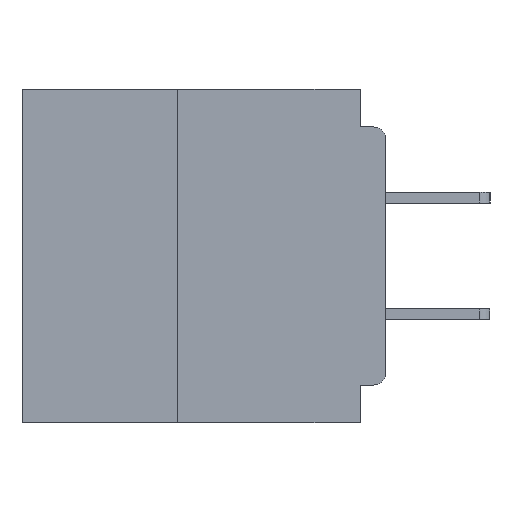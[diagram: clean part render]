
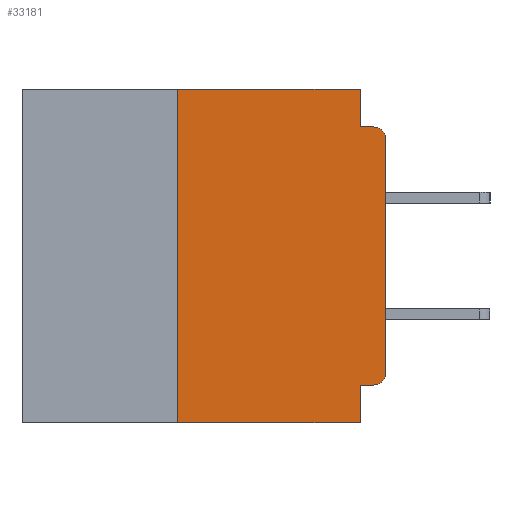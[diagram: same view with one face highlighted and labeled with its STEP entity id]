
A CAD part, left-side view. The second image highlights one B-rep face of the part: STEP entity #33181.
In plain terms, the highlighted planar face has unit normal (-1, 0, 0).
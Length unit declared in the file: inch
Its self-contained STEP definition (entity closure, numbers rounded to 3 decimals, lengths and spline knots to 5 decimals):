
#169 = CARTESIAN_POINT ( 'NONE',  ( 0., 0.437, 0. ) ) ;
#659 = CARTESIAN_POINT ( 'NONE',  ( 0., 0.015, -0.34 ) ) ;
#761 = ORIENTED_EDGE ( 'NONE', *, *, #18441, .F. ) ;
#800 = DIRECTION ( 'NONE',  ( 0., -1., 0. ) ) ;
#877 = VECTOR ( 'NONE', #6855, 39.37008 ) ;
#1191 = VECTOR ( 'NONE', #8662, 39.37008 ) ;
#1394 = LINE ( 'NONE', #33874, #30049 ) ;
#1563 = ORIENTED_EDGE ( 'NONE', *, *, #8156, .F. ) ;
#1566 = CARTESIAN_POINT ( 'NONE',  ( 0., 0.25, 0. ) ) ;
#2756 = CARTESIAN_POINT ( 'NONE',  ( 0., 0.031, 0. ) ) ;
#3075 = DIRECTION ( 'NONE',  ( 0., 0., -1. ) ) ;
#3431 = VECTOR ( 'NONE', #13379, 39.37008 ) ;
#3552 = DIRECTION ( 'NONE',  ( 0., 0., -1. ) ) ;
#4221 = VERTEX_POINT ( 'NONE', #32813 ) ;
#5037 = VERTEX_POINT ( 'NONE', #6826 ) ;
#5490 = CARTESIAN_POINT ( 'NONE',  ( 0., 0., -0.045 ) ) ;
#5972 = CARTESIAN_POINT ( 'NONE',  ( 0., 0.437, 0. ) ) ;
#6091 = DIRECTION ( 'NONE',  ( 0., -1., 0. ) ) ;
#6714 = LINE ( 'NONE', #35577, #28850 ) ;
#6826 = CARTESIAN_POINT ( 'NONE',  ( 0., 0., -0.34 ) ) ;
#6832 = ORIENTED_EDGE ( 'NONE', *, *, #22247, .T. ) ;
#6855 = DIRECTION ( 'NONE',  ( 0., 0., -1. ) ) ;
#7429 = CARTESIAN_POINT ( 'NONE',  ( 0., 0.015, -0.06 ) ) ;
#7729 = EDGE_LOOP ( 'NONE', ( #24704, #33731, #17093, #23660, #1563, #24869, #12643, #761, #22183, #6832 ) ) ;
#8156 = EDGE_CURVE ( 'NONE', #14080, #24318, #12377, .T. ) ;
#8567 = PLANE ( 'NONE',  #17278 ) ;
#8662 = DIRECTION ( 'NONE',  ( 0., 0., 1. ) ) ;
#9580 = CARTESIAN_POINT ( 'NONE',  ( 0., 0.031, -0.4 ) ) ;
#10043 = CARTESIAN_POINT ( 'NONE',  ( 0., 0.031, -0.4 ) ) ;
#10247 = DIRECTION ( 'NONE',  ( 0., 0., -1. ) ) ;
#11178 = CARTESIAN_POINT ( 'NONE',  ( 0., 0.015, -0.355 ) ) ;
#11506 = VERTEX_POINT ( 'NONE', #15536 ) ;
#11564 = VERTEX_POINT ( 'NONE', #26868 ) ;
#11615 = VECTOR ( 'NONE', #16721, 39.37008 ) ;
#12377 = LINE ( 'NONE', #5972, #18980 ) ;
#12612 = LINE ( 'NONE', #29885, #3431 ) ;
#12643 = ORIENTED_EDGE ( 'NONE', *, *, #27583, .T. ) ;
#13379 = DIRECTION ( 'NONE',  ( 0., 1., 0. ) ) ;
#13423 = VERTEX_POINT ( 'NONE', #10043 ) ;
#14080 = VERTEX_POINT ( 'NONE', #1566 ) ;
#15536 = CARTESIAN_POINT ( 'NONE',  ( 0., 0.031, -0.045 ) ) ;
#15836 = LINE ( 'NONE', #9580, #877 ) ;
#16721 = DIRECTION ( 'NONE',  ( 0., 0., -1. ) ) ;
#16782 = DIRECTION ( 'NONE',  ( 0., -1., 0. ) ) ;
#17027 = LINE ( 'NONE', #22579, #1191 ) ;
#17093 = ORIENTED_EDGE ( 'NONE', *, *, #17564, .F. ) ;
#17278 = AXIS2_PLACEMENT_3D ( 'NONE', #169, #19819, #3075 ) ;
#17564 = EDGE_CURVE ( 'NONE', #11506, #20044, #29651, .T. ) ;
#17688 = VERTEX_POINT ( 'NONE', #31086 ) ;
#17907 = CIRCLE ( 'NONE', #30913, 0.015 ) ;
#18441 = EDGE_CURVE ( 'NONE', #17688, #13423, #15836, .T. ) ;
#18980 = VECTOR ( 'NONE', #6091, 39.37008 ) ;
#19254 = CIRCLE ( 'NONE', #30952, 0.015 ) ;
#19414 = DIRECTION ( 'NONE',  ( 0., 0., 1. ) ) ;
#19819 = DIRECTION ( 'NONE',  ( 1., 0., 0. ) ) ;
#20044 = VERTEX_POINT ( 'NONE', #23678 ) ;
#20281 = DIRECTION ( 'NONE',  ( -1., 0., 0. ) ) ;
#20860 = CARTESIAN_POINT ( 'NONE',  ( 0., 0.031, 0. ) ) ;
#22183 = ORIENTED_EDGE ( 'NONE', *, *, #34793, .F. ) ;
#22247 = EDGE_CURVE ( 'NONE', #31831, #5037, #19254, .T. ) ;
#22579 = CARTESIAN_POINT ( 'NONE',  ( 0., 0., 0. ) ) ;
#23660 = ORIENTED_EDGE ( 'NONE', *, *, #30603, .F. ) ;
#23678 = CARTESIAN_POINT ( 'NONE',  ( 0., 0.015, -0.045 ) ) ;
#24101 = EDGE_CURVE ( 'NONE', #5037, #11564, #17027, .T. ) ;
#24318 = VERTEX_POINT ( 'NONE', #20860 ) ;
#24704 = ORIENTED_EDGE ( 'NONE', *, *, #24101, .T. ) ;
#24869 = ORIENTED_EDGE ( 'NONE', *, *, #31775, .F. ) ;
#26868 = CARTESIAN_POINT ( 'NONE',  ( 0., 0., -0.06 ) ) ;
#26884 = DIRECTION ( 'NONE',  ( -1., 0., 0. ) ) ;
#27583 = EDGE_CURVE ( 'NONE', #4221, #13423, #1394, .T. ) ;
#27985 = VECTOR ( 'NONE', #16782, 39.37008 ) ;
#28850 = VECTOR ( 'NONE', #19414, 39.37008 ) ;
#29594 = FACE_OUTER_BOUND ( 'NONE', #7729, .T. ) ;
#29637 = EDGE_CURVE ( 'NONE', #11564, #20044, #17907, .T. ) ;
#29651 = LINE ( 'NONE', #5490, #27985 ) ;
#29885 = CARTESIAN_POINT ( 'NONE',  ( 0., 0., -0.355 ) ) ;
#30049 = VECTOR ( 'NONE', #800, 39.37008 ) ;
#30603 = EDGE_CURVE ( 'NONE', #24318, #11506, #33519, .T. ) ;
#30913 = AXIS2_PLACEMENT_3D ( 'NONE', #7429, #26884, #10247 ) ;
#30952 = AXIS2_PLACEMENT_3D ( 'NONE', #659, #20281, #3552 ) ;
#31086 = CARTESIAN_POINT ( 'NONE',  ( 0., 0.031, -0.355 ) ) ;
#31775 = EDGE_CURVE ( 'NONE', #4221, #14080, #6714, .T. ) ;
#31831 = VERTEX_POINT ( 'NONE', #11178 ) ;
#32813 = CARTESIAN_POINT ( 'NONE',  ( 0., 0.25, -0.4 ) ) ;
#33181 = ADVANCED_FACE ( 'NONE', ( #29594 ), #8567, .F. ) ;
#33519 = LINE ( 'NONE', #2756, #11615 ) ;
#33731 = ORIENTED_EDGE ( 'NONE', *, *, #29637, .T. ) ;
#33874 = CARTESIAN_POINT ( 'NONE',  ( 0., 0.437, -0.4 ) ) ;
#34793 = EDGE_CURVE ( 'NONE', #31831, #17688, #12612, .T. ) ;
#35577 = CARTESIAN_POINT ( 'NONE',  ( 0., 0.25, -0.4 ) ) ;
